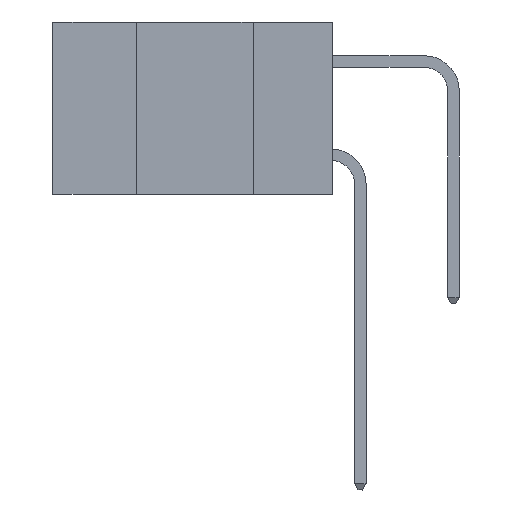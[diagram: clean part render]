
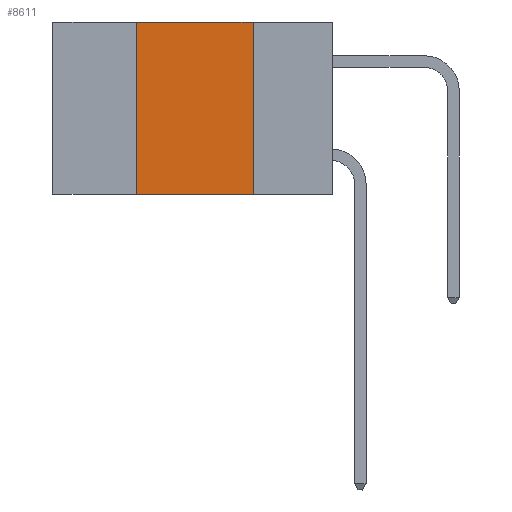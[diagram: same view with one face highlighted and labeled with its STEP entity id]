
A CAD part, left-side view. The second image highlights one B-rep face of the part: STEP entity #8611.
In plain terms, the highlighted planar face has unit normal (-1, 0, 0).
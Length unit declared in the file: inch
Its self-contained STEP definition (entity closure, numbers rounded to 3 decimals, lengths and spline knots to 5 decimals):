
#133 = DIRECTION ( 'NONE',  ( 0., 0., 1. ) ) ;
#818 = VERTEX_POINT ( 'NONE', #6049 ) ;
#924 = DIRECTION ( 'NONE',  ( 0., -1., 0. ) ) ;
#954 = CARTESIAN_POINT ( 'NONE',  ( 0., 0.42, -0.37 ) ) ;
#1308 = ORIENTED_EDGE ( 'NONE', *, *, #16334, .T. ) ;
#1334 = PLANE ( 'NONE',  #16115 ) ;
#2596 = CARTESIAN_POINT ( 'NONE',  ( 0., 0.17, 0. ) ) ;
#3097 = CARTESIAN_POINT ( 'NONE',  ( 0., 0.6, 0. ) ) ;
#3234 = LINE ( 'NONE', #2596, #20364 ) ;
#3375 = LINE ( 'NONE', #12092, #21054 ) ;
#3686 = CARTESIAN_POINT ( 'NONE',  ( 0., 0.42, 0. ) ) ;
#4046 = VERTEX_POINT ( 'NONE', #3686 ) ;
#4449 = FACE_OUTER_BOUND ( 'NONE', #6127, .T. ) ;
#4814 = DIRECTION ( 'NONE',  ( 1., 0., 0. ) ) ;
#6049 = CARTESIAN_POINT ( 'NONE',  ( 0., 0.17, 0. ) ) ;
#6127 = EDGE_LOOP ( 'NONE', ( #21487, #12868, #16646, #1308 ) ) ;
#7760 = DIRECTION ( 'NONE',  ( 0., 0., -1. ) ) ;
#7836 = CARTESIAN_POINT ( 'NONE',  ( 0., 0.6, 0. ) ) ;
#8611 = ADVANCED_FACE ( 'NONE', ( #4449 ), #1334, .F. ) ;
#9724 = EDGE_CURVE ( 'NONE', #4046, #818, #13012, .T. ) ;
#10424 = DIRECTION ( 'NONE',  ( 0., -1., 0. ) ) ;
#12092 = CARTESIAN_POINT ( 'NONE',  ( 0., 0.42, 0. ) ) ;
#12177 = VERTEX_POINT ( 'NONE', #13941 ) ;
#12868 = ORIENTED_EDGE ( 'NONE', *, *, #9724, .F. ) ;
#13012 = LINE ( 'NONE', #7836, #21587 ) ;
#13941 = CARTESIAN_POINT ( 'NONE',  ( 0., 0.17, -0.37 ) ) ;
#14180 = LINE ( 'NONE', #20765, #19280 ) ;
#14672 = EDGE_CURVE ( 'NONE', #818, #12177, #3234, .T. ) ;
#16115 = AXIS2_PLACEMENT_3D ( 'NONE', #3097, #4814, #16835 ) ;
#16334 = EDGE_CURVE ( 'NONE', #16628, #12177, #14180, .T. ) ;
#16628 = VERTEX_POINT ( 'NONE', #954 ) ;
#16646 = ORIENTED_EDGE ( 'NONE', *, *, #18203, .F. ) ;
#16835 = DIRECTION ( 'NONE',  ( 0., 0., -1. ) ) ;
#18203 = EDGE_CURVE ( 'NONE', #16628, #4046, #3375, .T. ) ;
#19280 = VECTOR ( 'NONE', #10424, 39.37008 ) ;
#20364 = VECTOR ( 'NONE', #7760, 39.37008 ) ;
#20765 = CARTESIAN_POINT ( 'NONE',  ( 0., 0.6, -0.37 ) ) ;
#21054 = VECTOR ( 'NONE', #133, 39.37008 ) ;
#21487 = ORIENTED_EDGE ( 'NONE', *, *, #14672, .F. ) ;
#21587 = VECTOR ( 'NONE', #924, 39.37008 ) ;
